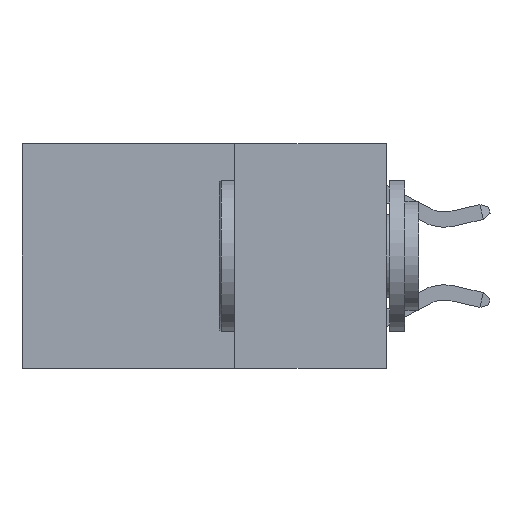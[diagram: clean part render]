
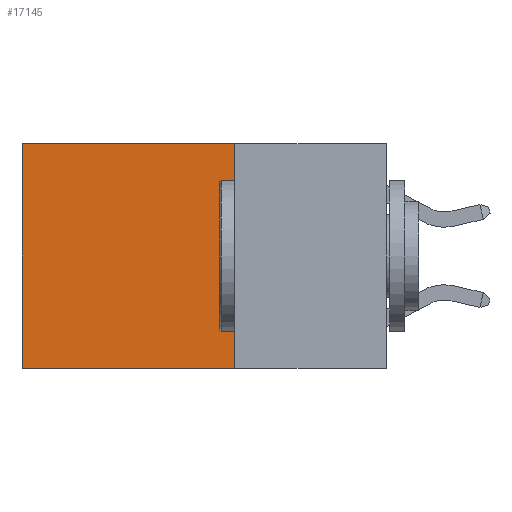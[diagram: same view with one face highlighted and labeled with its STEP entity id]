
A CAD part, left-side view. The second image highlights one B-rep face of the part: STEP entity #17145.
In plain terms, the highlighted planar face has unit normal (-1, 0, 0).
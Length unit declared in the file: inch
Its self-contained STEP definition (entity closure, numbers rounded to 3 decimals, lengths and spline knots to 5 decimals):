
#47 = AXIS2_PLACEMENT_3D ( 'NONE', #11191, #12517, #4307 ) ;
#63 = VECTOR ( 'NONE', #4079, 39.37008 ) ;
#281 = DIRECTION ( 'NONE',  ( 0., 0., -1. ) ) ;
#394 = VERTEX_POINT ( 'NONE', #13402 ) ;
#801 = VECTOR ( 'NONE', #12239, 39.37008 ) ;
#1091 = DIRECTION ( 'NONE',  ( 0., 1., 0. ) ) ;
#2112 = EDGE_CURVE ( 'NONE', #3787, #3882, #15557, .T. ) ;
#3294 = EDGE_LOOP ( 'NONE', ( #10837, #7659, #11249, #8104 ) ) ;
#3787 = VERTEX_POINT ( 'NONE', #14852 ) ;
#3882 = VERTEX_POINT ( 'NONE', #17724 ) ;
#3990 = VECTOR ( 'NONE', #281, 39.37008 ) ;
#4079 = DIRECTION ( 'NONE',  ( 0., 1., 0. ) ) ;
#4144 = EDGE_CURVE ( 'NONE', #12254, #394, #14871, .T. ) ;
#4307 = DIRECTION ( 'NONE',  ( 0., 0., -1. ) ) ;
#7659 = ORIENTED_EDGE ( 'NONE', *, *, #9351, .F. ) ;
#8104 = ORIENTED_EDGE ( 'NONE', *, *, #10951, .T. ) ;
#8193 = CARTESIAN_POINT ( 'NONE',  ( 0.2625, 0.25, 0. ) ) ;
#9351 = EDGE_CURVE ( 'NONE', #3882, #394, #15004, .T. ) ;
#10308 = CARTESIAN_POINT ( 'NONE',  ( 0.2625, 0.6, 0. ) ) ;
#10837 = ORIENTED_EDGE ( 'NONE', *, *, #4144, .T. ) ;
#10951 = EDGE_CURVE ( 'NONE', #3787, #12254, #14537, .T. ) ;
#11191 = CARTESIAN_POINT ( 'NONE',  ( 0.2625, 0.25, 0. ) ) ;
#11249 = ORIENTED_EDGE ( 'NONE', *, *, #2112, .F. ) ;
#12239 = DIRECTION ( 'NONE',  ( 0., 0., -1. ) ) ;
#12254 = VERTEX_POINT ( 'NONE', #17251 ) ;
#12321 = CARTESIAN_POINT ( 'NONE',  ( 0.2625, 0.25, 0. ) ) ;
#12412 = PLANE ( 'NONE',  #47 ) ;
#12517 = DIRECTION ( 'NONE',  ( 1., 0., 0. ) ) ;
#13402 = CARTESIAN_POINT ( 'NONE',  ( 0.2625, 0.6, -0.37 ) ) ;
#14184 = VECTOR ( 'NONE', #1091, 39.37008 ) ;
#14537 = LINE ( 'NONE', #12321, #63 ) ;
#14852 = CARTESIAN_POINT ( 'NONE',  ( 0.2625, 0.25, 0. ) ) ;
#14871 = LINE ( 'NONE', #10308, #3990 ) ;
#15004 = LINE ( 'NONE', #17562, #14184 ) ;
#15557 = LINE ( 'NONE', #8193, #801 ) ;
#17145 = ADVANCED_FACE ( 'NONE', ( #17221 ), #12412, .F. ) ;
#17221 = FACE_OUTER_BOUND ( 'NONE', #3294, .T. ) ;
#17251 = CARTESIAN_POINT ( 'NONE',  ( 0.2625, 0.6, 0. ) ) ;
#17562 = CARTESIAN_POINT ( 'NONE',  ( 0.2625, 0.25, -0.37 ) ) ;
#17724 = CARTESIAN_POINT ( 'NONE',  ( 0.2625, 0.25, -0.37 ) ) ;
